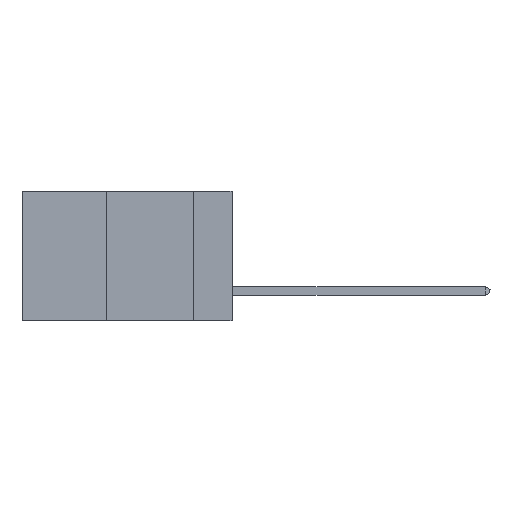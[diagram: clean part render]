
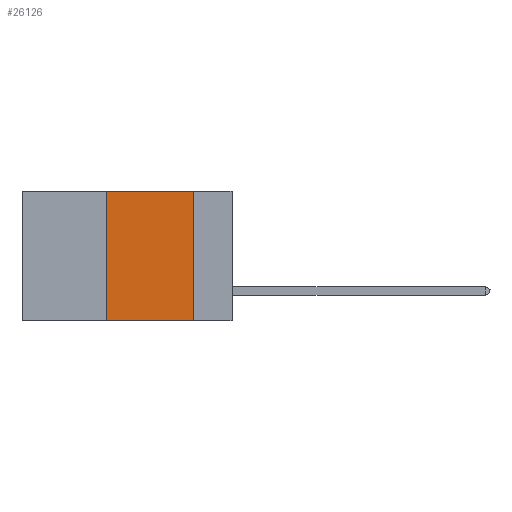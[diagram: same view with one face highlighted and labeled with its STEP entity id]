
A CAD part, left-side view. The second image highlights one B-rep face of the part: STEP entity #26126.
In plain terms, the highlighted planar face has unit normal (-1, 0, 0).
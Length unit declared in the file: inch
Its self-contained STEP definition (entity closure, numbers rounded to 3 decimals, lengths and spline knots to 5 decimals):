
#217 = CARTESIAN_POINT ( 'NONE',  ( 0., 0.6, -0.37 ) ) ;
#821 = VERTEX_POINT ( 'NONE', #19417 ) ;
#3227 = EDGE_LOOP ( 'NONE', ( #28411, #9958, #22530, #22375 ) ) ;
#3871 = CARTESIAN_POINT ( 'NONE',  ( 0., 0.6, 0. ) ) ;
#4327 = VERTEX_POINT ( 'NONE', #28700 ) ;
#6637 = VECTOR ( 'NONE', #13784, 39.37008 ) ;
#7701 = CARTESIAN_POINT ( 'NONE',  ( 0., 0.11, 0. ) ) ;
#8535 = EDGE_CURVE ( 'NONE', #41533, #25560, #10470, .T. ) ;
#9958 = ORIENTED_EDGE ( 'NONE', *, *, #30185, .F. ) ;
#10470 = LINE ( 'NONE', #217, #12106 ) ;
#10635 = DIRECTION ( 'NONE',  ( 0., 0., 1. ) ) ;
#12106 = VECTOR ( 'NONE', #20837, 39.37008 ) ;
#13784 = DIRECTION ( 'NONE',  ( 0., -1., 0. ) ) ;
#16196 = CARTESIAN_POINT ( 'NONE',  ( 0., 0.36, 0. ) ) ;
#16543 = LINE ( 'NONE', #27881, #6637 ) ;
#19409 = FACE_OUTER_BOUND ( 'NONE', #3227, .T. ) ;
#19417 = CARTESIAN_POINT ( 'NONE',  ( 0., 0.11, 0. ) ) ;
#20059 = LINE ( 'NONE', #7701, #30079 ) ;
#20395 = EDGE_CURVE ( 'NONE', #821, #25560, #20059, .T. ) ;
#20837 = DIRECTION ( 'NONE',  ( 0., -1., 0. ) ) ;
#22375 = ORIENTED_EDGE ( 'NONE', *, *, #8535, .T. ) ;
#22530 = ORIENTED_EDGE ( 'NONE', *, *, #24348, .F. ) ;
#24348 = EDGE_CURVE ( 'NONE', #41533, #4327, #27958, .T. ) ;
#25442 = CARTESIAN_POINT ( 'NONE',  ( 0., 0.11, -0.37 ) ) ;
#25560 = VERTEX_POINT ( 'NONE', #25442 ) ;
#26126 = ADVANCED_FACE ( 'NONE', ( #19409 ), #42820, .F. ) ;
#27881 = CARTESIAN_POINT ( 'NONE',  ( 0., 0.6, 0. ) ) ;
#27958 = LINE ( 'NONE', #16196, #32463 ) ;
#28411 = ORIENTED_EDGE ( 'NONE', *, *, #20395, .F. ) ;
#28700 = CARTESIAN_POINT ( 'NONE',  ( 0., 0.36, 0. ) ) ;
#30079 = VECTOR ( 'NONE', #43676, 39.37008 ) ;
#30185 = EDGE_CURVE ( 'NONE', #4327, #821, #16543, .T. ) ;
#32266 = DIRECTION ( 'NONE',  ( 0., 0., -1. ) ) ;
#32463 = VECTOR ( 'NONE', #10635, 39.37008 ) ;
#41533 = VERTEX_POINT ( 'NONE', #41728 ) ;
#41728 = CARTESIAN_POINT ( 'NONE',  ( 0., 0.36, -0.37 ) ) ;
#42820 = PLANE ( 'NONE',  #43637 ) ;
#42965 = DIRECTION ( 'NONE',  ( 1., 0., 0. ) ) ;
#43637 = AXIS2_PLACEMENT_3D ( 'NONE', #3871, #42965, #32266 ) ;
#43676 = DIRECTION ( 'NONE',  ( 0., 0., -1. ) ) ;
